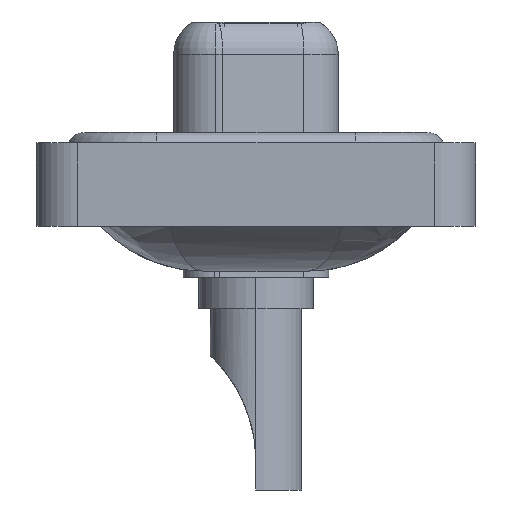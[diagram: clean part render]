
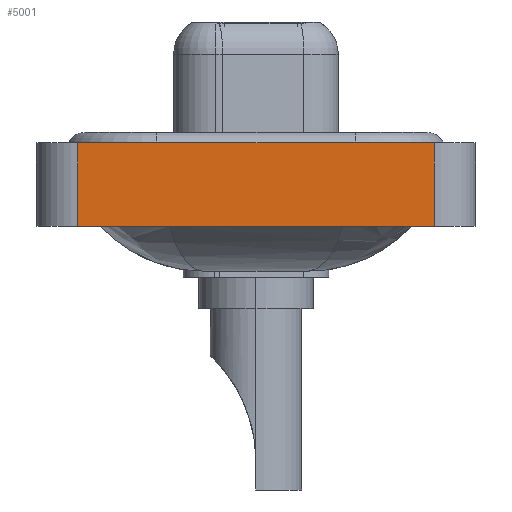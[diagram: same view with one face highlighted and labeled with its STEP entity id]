
A CAD part, left-side view. The second image highlights one B-rep face of the part: STEP entity #5001.
In plain terms, the highlighted planar face has unit normal (-1, 0, 0).
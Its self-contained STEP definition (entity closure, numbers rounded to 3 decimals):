
#80 = CARTESIAN_POINT ( 'NONE',  ( -7.35, -8.55, 0.4 ) ) ;
#82 = DIRECTION ( 'NONE',  ( 0., 0., 1. ) ) ;
#341 = LINE ( 'NONE', #14487, #1137 ) ;
#478 = EDGE_LOOP ( 'NONE', ( #11625, #4656, #9909, #14299 ) ) ;
#1137 = VECTOR ( 'NONE', #3016, 1000. ) ;
#1187 = EDGE_CURVE ( 'NONE', #12310, #12974, #341, .T. ) ;
#1638 = VECTOR ( 'NONE', #10269, 1000. ) ;
#1713 = DIRECTION ( 'NONE',  ( 0., -1., 0. ) ) ;
#2311 = EDGE_CURVE ( 'NONE', #12974, #3647, #15163, .T. ) ;
#2472 = LINE ( 'NONE', #2551, #1638 ) ;
#2551 = CARTESIAN_POINT ( 'NONE',  ( -7.35, 8.55, -3.6 ) ) ;
#2964 = LINE ( 'NONE', #12015, #12223 ) ;
#3016 = DIRECTION ( 'NONE',  ( 0., -1., 0. ) ) ;
#3647 = VERTEX_POINT ( 'NONE', #80 ) ;
#3929 = EDGE_CURVE ( 'NONE', #12310, #7816, #2472, .T. ) ;
#4376 = VECTOR ( 'NONE', #11331, 1000. ) ;
#4656 = ORIENTED_EDGE ( 'NONE', *, *, #9765, .F. ) ;
#5001 = ADVANCED_FACE ( 'NONE', ( #7851 ), #7678, .T. ) ;
#6571 = CARTESIAN_POINT ( 'NONE',  ( -7.35, 8.55, -3.6 ) ) ;
#7678 = PLANE ( 'NONE',  #8319 ) ;
#7816 = VERTEX_POINT ( 'NONE', #10045 ) ;
#7851 = FACE_OUTER_BOUND ( 'NONE', #478, .T. ) ;
#8319 = AXIS2_PLACEMENT_3D ( 'NONE', #14318, #11724, #82 ) ;
#8384 = CARTESIAN_POINT ( 'NONE',  ( -7.35, -8.55, -3.6 ) ) ;
#9765 = EDGE_CURVE ( 'NONE', #7816, #3647, #2964, .T. ) ;
#9909 = ORIENTED_EDGE ( 'NONE', *, *, #3929, .F. ) ;
#10045 = CARTESIAN_POINT ( 'NONE',  ( -7.35, 8.55, 0.4 ) ) ;
#10269 = DIRECTION ( 'NONE',  ( 0., 0., 1. ) ) ;
#11331 = DIRECTION ( 'NONE',  ( 0., 0., 1. ) ) ;
#11625 = ORIENTED_EDGE ( 'NONE', *, *, #2311, .T. ) ;
#11724 = DIRECTION ( 'NONE',  ( -1., 0., 0. ) ) ;
#12015 = CARTESIAN_POINT ( 'NONE',  ( -7.35, -8.55, 0.4 ) ) ;
#12223 = VECTOR ( 'NONE', #1713, 1000. ) ;
#12310 = VERTEX_POINT ( 'NONE', #6571 ) ;
#12501 = CARTESIAN_POINT ( 'NONE',  ( -7.35, -8.55, -3.6 ) ) ;
#12974 = VERTEX_POINT ( 'NONE', #8384 ) ;
#14299 = ORIENTED_EDGE ( 'NONE', *, *, #1187, .T. ) ;
#14318 = CARTESIAN_POINT ( 'NONE',  ( -7.35, -8.55, -3.6 ) ) ;
#14487 = CARTESIAN_POINT ( 'NONE',  ( -7.35, -8.55, -3.6 ) ) ;
#15163 = LINE ( 'NONE', #12501, #4376 ) ;
